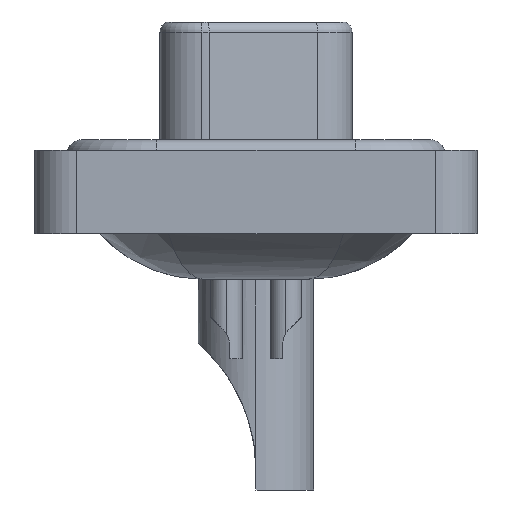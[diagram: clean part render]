
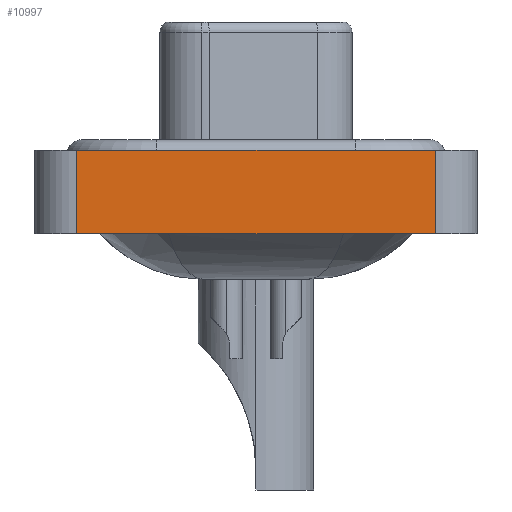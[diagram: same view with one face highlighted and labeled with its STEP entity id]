
A CAD part, left-side view. The second image highlights one B-rep face of the part: STEP entity #10997.
In plain terms, the highlighted planar face has unit normal (-1, 0, 0).
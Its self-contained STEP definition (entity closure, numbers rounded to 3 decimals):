
#31 = CARTESIAN_POINT ( 'NONE',  ( -7.25, 8.55, -3.6 ) ) ;
#1383 = LINE ( 'NONE', #6965, #11089 ) ;
#2266 = ORIENTED_EDGE ( 'NONE', *, *, #13674, .T. ) ;
#2941 = CARTESIAN_POINT ( 'NONE',  ( -7.25, -8.55, -3.6 ) ) ;
#3153 = VERTEX_POINT ( 'NONE', #16997 ) ;
#3441 = LINE ( 'NONE', #11593, #10071 ) ;
#4311 = FACE_OUTER_BOUND ( 'NONE', #11378, .T. ) ;
#5724 = CARTESIAN_POINT ( 'NONE',  ( -7.25, -8.55, -3.6 ) ) ;
#6283 = DIRECTION ( 'NONE',  ( 0., -1., 0. ) ) ;
#6698 = DIRECTION ( 'NONE',  ( 0., 0., 1. ) ) ;
#6965 = CARTESIAN_POINT ( 'NONE',  ( -7.25, 8.55, -3.6 ) ) ;
#7062 = VECTOR ( 'NONE', #16838, 1000. ) ;
#7394 = AXIS2_PLACEMENT_3D ( 'NONE', #2941, #8513, #6698 ) ;
#7957 = CARTESIAN_POINT ( 'NONE',  ( -7.25, -8.55, -3.6 ) ) ;
#7970 = VERTEX_POINT ( 'NONE', #7957 ) ;
#8179 = EDGE_CURVE ( 'NONE', #3153, #11798, #8580, .T. ) ;
#8310 = DIRECTION ( 'NONE',  ( 0., -1., 0. ) ) ;
#8513 = DIRECTION ( 'NONE',  ( -1., 0., 0. ) ) ;
#8580 = LINE ( 'NONE', #15668, #16535 ) ;
#8692 = EDGE_CURVE ( 'NONE', #15062, #7970, #3441, .T. ) ;
#9154 = ORIENTED_EDGE ( 'NONE', *, *, #8179, .F. ) ;
#9887 = PLANE ( 'NONE',  #7394 ) ;
#10071 = VECTOR ( 'NONE', #6283, 1000. ) ;
#10997 = ADVANCED_FACE ( 'NONE', ( #4311 ), #9887, .T. ) ;
#11089 = VECTOR ( 'NONE', #12660, 1000. ) ;
#11378 = EDGE_LOOP ( 'NONE', ( #2266, #9154, #13368, #16196 ) ) ;
#11593 = CARTESIAN_POINT ( 'NONE',  ( -7.25, -8.55, -3.6 ) ) ;
#11798 = VERTEX_POINT ( 'NONE', #13896 ) ;
#12660 = DIRECTION ( 'NONE',  ( 0., 0., 1. ) ) ;
#13368 = ORIENTED_EDGE ( 'NONE', *, *, #15459, .F. ) ;
#13674 = EDGE_CURVE ( 'NONE', #7970, #11798, #13784, .T. ) ;
#13784 = LINE ( 'NONE', #5724, #7062 ) ;
#13896 = CARTESIAN_POINT ( 'NONE',  ( -7.25, -8.55, 0.4 ) ) ;
#15062 = VERTEX_POINT ( 'NONE', #31 ) ;
#15459 = EDGE_CURVE ( 'NONE', #15062, #3153, #1383, .T. ) ;
#15668 = CARTESIAN_POINT ( 'NONE',  ( -7.25, -8.55, 0.4 ) ) ;
#16196 = ORIENTED_EDGE ( 'NONE', *, *, #8692, .T. ) ;
#16535 = VECTOR ( 'NONE', #8310, 1000. ) ;
#16838 = DIRECTION ( 'NONE',  ( 0., 0., 1. ) ) ;
#16997 = CARTESIAN_POINT ( 'NONE',  ( -7.25, 8.55, 0.4 ) ) ;
